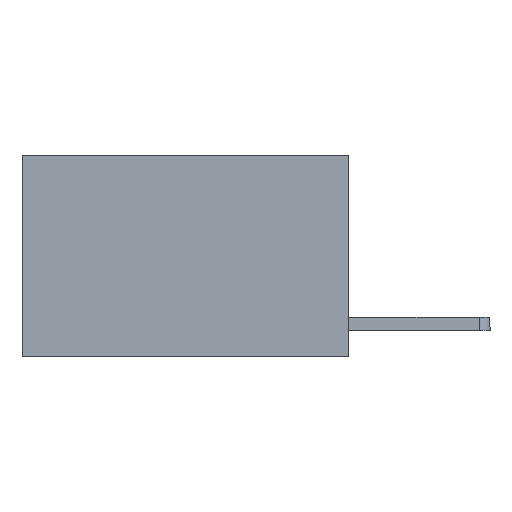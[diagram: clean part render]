
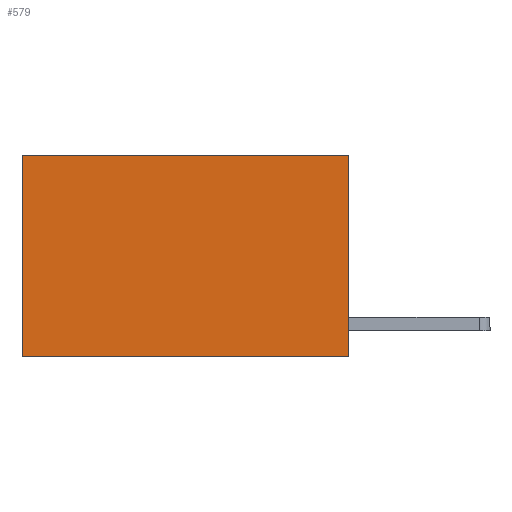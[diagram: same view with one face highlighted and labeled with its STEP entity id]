
A CAD part, left-side view. The second image highlights one B-rep face of the part: STEP entity #579.
In plain terms, the highlighted planar face has unit normal (-1, 0, 0).
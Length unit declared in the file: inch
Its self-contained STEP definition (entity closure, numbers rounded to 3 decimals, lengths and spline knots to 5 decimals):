
#1 = DIRECTION ( 'NONE',  ( 0., 0., -1. ) ) ;
#579 = ADVANCED_FACE ( 'NONE', ( #2317 ), #1550, .F. ) ;
#778 = DIRECTION ( 'NONE',  ( 1., 0., 0. ) ) ;
#910 = VECTOR ( 'NONE', #8265, 39.37008 ) ;
#977 = ORIENTED_EDGE ( 'NONE', *, *, #1972, .T. ) ;
#1016 = VERTEX_POINT ( 'NONE', #3978 ) ;
#1082 = LINE ( 'NONE', #5181, #910 ) ;
#1135 = CARTESIAN_POINT ( 'NONE',  ( 0.2625, 0.6, 0. ) ) ;
#1416 = ORIENTED_EDGE ( 'NONE', *, *, #5505, .F. ) ;
#1550 = PLANE ( 'NONE',  #8033 ) ;
#1972 = EDGE_CURVE ( 'NONE', #10019, #9652, #5715, .T. ) ;
#2095 = CARTESIAN_POINT ( 'NONE',  ( 0.2625, 0., 0. ) ) ;
#2203 = LINE ( 'NONE', #3891, #9382 ) ;
#2317 = FACE_OUTER_BOUND ( 'NONE', #7689, .T. ) ;
#2556 = EDGE_CURVE ( 'NONE', #1016, #6149, #9360, .T. ) ;
#2973 = DIRECTION ( 'NONE',  ( 0., 0., -1. ) ) ;
#3359 = CARTESIAN_POINT ( 'NONE',  ( 0.2625, 0., -0.37 ) ) ;
#3891 = CARTESIAN_POINT ( 'NONE',  ( 0.2625, 0., -0.37 ) ) ;
#3978 = CARTESIAN_POINT ( 'NONE',  ( 0.2625, 0., 0. ) ) ;
#4123 = EDGE_CURVE ( 'NONE', #1016, #10019, #1082, .T. ) ;
#5041 = VECTOR ( 'NONE', #2973, 39.37008 ) ;
#5181 = CARTESIAN_POINT ( 'NONE',  ( 0.2625, 0., 0. ) ) ;
#5505 = EDGE_CURVE ( 'NONE', #6149, #9652, #2203, .T. ) ;
#5542 = VECTOR ( 'NONE', #6581, 39.37008 ) ;
#5715 = LINE ( 'NONE', #1135, #5542 ) ;
#6149 = VERTEX_POINT ( 'NONE', #3359 ) ;
#6247 = CARTESIAN_POINT ( 'NONE',  ( 0.2625, 0.6, 0. ) ) ;
#6581 = DIRECTION ( 'NONE',  ( 0., 0., -1. ) ) ;
#6788 = ORIENTED_EDGE ( 'NONE', *, *, #2556, .F. ) ;
#7689 = EDGE_LOOP ( 'NONE', ( #977, #1416, #6788, #9561 ) ) ;
#7716 = CARTESIAN_POINT ( 'NONE',  ( 0.2625, 0.6, -0.37 ) ) ;
#7820 = CARTESIAN_POINT ( 'NONE',  ( 0.2625, 0., 0. ) ) ;
#8033 = AXIS2_PLACEMENT_3D ( 'NONE', #7820, #778, #1 ) ;
#8265 = DIRECTION ( 'NONE',  ( 0., 1., 0. ) ) ;
#8422 = DIRECTION ( 'NONE',  ( 0., 1., 0. ) ) ;
#9360 = LINE ( 'NONE', #2095, #5041 ) ;
#9382 = VECTOR ( 'NONE', #8422, 39.37008 ) ;
#9561 = ORIENTED_EDGE ( 'NONE', *, *, #4123, .T. ) ;
#9652 = VERTEX_POINT ( 'NONE', #7716 ) ;
#10019 = VERTEX_POINT ( 'NONE', #6247 ) ;
